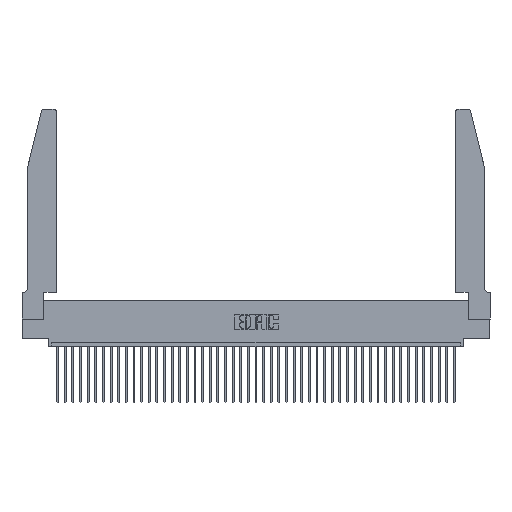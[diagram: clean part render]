
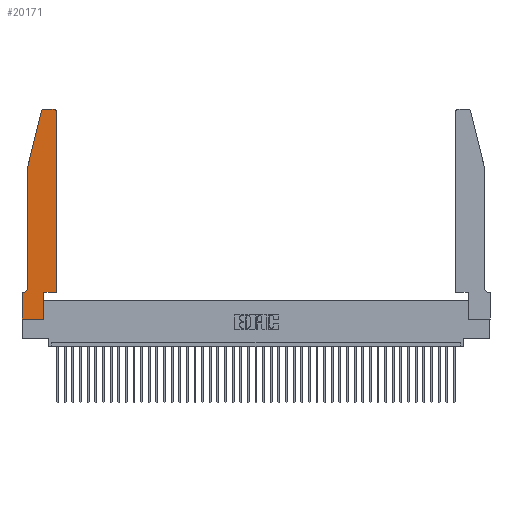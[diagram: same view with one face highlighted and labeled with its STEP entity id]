
A CAD part, top view. The second image highlights one B-rep face of the part: STEP entity #20171.
In plain terms, the highlighted planar face has unit normal (0, 0, 1).
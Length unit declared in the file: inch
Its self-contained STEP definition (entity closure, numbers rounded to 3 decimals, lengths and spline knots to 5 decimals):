
#223 = CARTESIAN_POINT ( 'NONE',  ( 0.4205, 2.72, 0.37 ) ) ;
#619 = AXIS2_PLACEMENT_3D ( 'NONE', #31257, #7567, #41190 ) ;
#623 = ORIENTED_EDGE ( 'NONE', *, *, #8489, .T. ) ;
#880 = CARTESIAN_POINT ( 'NONE',  ( 0.4505, 0.35, 0.37 ) ) ;
#1090 = ORIENTED_EDGE ( 'NONE', *, *, #26192, .T. ) ;
#1239 = CARTESIAN_POINT ( 'NONE',  ( 0.4205, 2.75, 0.37 ) ) ;
#1270 = CARTESIAN_POINT ( 'NONE',  ( 0.284, 2.75, 0.37 ) ) ;
#1503 = VERTEX_POINT ( 'NONE', #7037 ) ;
#1797 = DIRECTION ( 'NONE',  ( 0., 0., 1. ) ) ;
#5428 = LINE ( 'NONE', #5480, #12282 ) ;
#5480 = CARTESIAN_POINT ( 'NONE',  ( 0.4505, 0.35, 0.37 ) ) ;
#5614 = VERTEX_POINT ( 'NONE', #9768 ) ;
#6310 = ORIENTED_EDGE ( 'NONE', *, *, #35478, .T. ) ;
#6558 = LINE ( 'NONE', #9406, #32181 ) ;
#7037 = CARTESIAN_POINT ( 'NONE',  ( 0., 0.35, 0.37 ) ) ;
#7567 = DIRECTION ( 'NONE',  ( 0., 0., -1. ) ) ;
#8362 = VERTEX_POINT ( 'NONE', #10703 ) ;
#8384 = DIRECTION ( 'NONE',  ( 0., 1., 0. ) ) ;
#8489 = EDGE_CURVE ( 'NONE', #17175, #11979, #5428, .T. ) ;
#9182 = EDGE_CURVE ( 'NONE', #5614, #41324, #26899, .T. ) ;
#9406 = CARTESIAN_POINT ( 'NONE',  ( 0.0755, 2., 0.37 ) ) ;
#9527 = LINE ( 'NONE', #24423, #42977 ) ;
#9768 = CARTESIAN_POINT ( 'NONE',  ( 0., 0., 0.37 ) ) ;
#10390 = VERTEX_POINT ( 'NONE', #1270 ) ;
#10703 = CARTESIAN_POINT ( 'NONE',  ( 0.4505, 2.72, 0.37 ) ) ;
#11257 = AXIS2_PLACEMENT_3D ( 'NONE', #16678, #16818, #20434 ) ;
#11530 = CARTESIAN_POINT ( 'NONE',  ( 0.25487, 2.72718, 0.37 ) ) ;
#11979 = VERTEX_POINT ( 'NONE', #29067 ) ;
#12216 = EDGE_CURVE ( 'NONE', #32223, #40770, #21927, .T. ) ;
#12282 = VECTOR ( 'NONE', #39114, 39.37008 ) ;
#12546 = VERTEX_POINT ( 'NONE', #33564 ) ;
#12661 = VERTEX_POINT ( 'NONE', #1239 ) ;
#12969 = ORIENTED_EDGE ( 'NONE', *, *, #9182, .T. ) ;
#13023 = CARTESIAN_POINT ( 'NONE',  ( 0.0755, 2., 0.37 ) ) ;
#13304 = PLANE ( 'NONE',  #11257 ) ;
#13798 = VERTEX_POINT ( 'NONE', #11530 ) ;
#13979 = FACE_OUTER_BOUND ( 'NONE', #34819, .T. ) ;
#14500 = ORIENTED_EDGE ( 'NONE', *, *, #36134, .T. ) ;
#15165 = CARTESIAN_POINT ( 'NONE',  ( 0.2865, 0.35, 0.37 ) ) ;
#15218 = ORIENTED_EDGE ( 'NONE', *, *, #26518, .T. ) ;
#16555 = DIRECTION ( 'NONE',  ( 1., 0., 0. ) ) ;
#16678 = CARTESIAN_POINT ( 'NONE',  ( 0., 0.35, 0.37 ) ) ;
#16818 = DIRECTION ( 'NONE',  ( 0., 0., 1. ) ) ;
#16928 = LINE ( 'NONE', #13023, #32581 ) ;
#17175 = VERTEX_POINT ( 'NONE', #19725 ) ;
#18486 = ORIENTED_EDGE ( 'NONE', *, *, #12216, .T. ) ;
#18670 = EDGE_CURVE ( 'NONE', #10390, #13798, #35825, .T. ) ;
#19725 = CARTESIAN_POINT ( 'NONE',  ( 0.2865, 0.35, 0.37 ) ) ;
#20171 = ADVANCED_FACE ( 'NONE', ( #13979 ), #13304, .T. ) ;
#20434 = DIRECTION ( 'NONE',  ( 1., 0., 0. ) ) ;
#21247 = ORIENTED_EDGE ( 'NONE', *, *, #32891, .T. ) ;
#21551 = DIRECTION ( 'NONE',  ( 0., 1., 0. ) ) ;
#21913 = VECTOR ( 'NONE', #25814, 39.37008 ) ;
#21927 = CIRCLE ( 'NONE', #619, 0.07 ) ;
#22358 = EDGE_CURVE ( 'NONE', #1503, #5614, #9527, .T. ) ;
#22671 = CARTESIAN_POINT ( 'NONE',  ( 0.0755, 0.42, 0.37 ) ) ;
#22992 = LINE ( 'NONE', #38913, #21913 ) ;
#24009 = LINE ( 'NONE', #39280, #36523 ) ;
#24423 = CARTESIAN_POINT ( 'NONE',  ( 0., 0., 0.37 ) ) ;
#24719 = EDGE_CURVE ( 'NONE', #40770, #1503, #22992, .T. ) ;
#25194 = VECTOR ( 'NONE', #8384, 39.37008 ) ;
#25288 = DIRECTION ( 'NONE',  ( 1., 0., 0. ) ) ;
#25814 = DIRECTION ( 'NONE',  ( -1., 0., 0. ) ) ;
#26192 = EDGE_CURVE ( 'NONE', #8362, #12661, #26679, .T. ) ;
#26518 = EDGE_CURVE ( 'NONE', #12661, #10390, #24009, .T. ) ;
#26641 = DIRECTION ( 'NONE',  ( 0., 0., 1. ) ) ;
#26679 = CIRCLE ( 'NONE', #35533, 0.03 ) ;
#26899 = LINE ( 'NONE', #28851, #35159 ) ;
#28851 = CARTESIAN_POINT ( 'NONE',  ( 0., 0., 0.37 ) ) ;
#29067 = CARTESIAN_POINT ( 'NONE',  ( 0.4505, 0.35, 0.37 ) ) ;
#30878 = LINE ( 'NONE', #15165, #25194 ) ;
#31257 = CARTESIAN_POINT ( 'NONE',  ( 0.0055, 0.42, 0.37 ) ) ;
#31733 = DIRECTION ( 'NONE',  ( 1., 0., 0. ) ) ;
#31855 = ORIENTED_EDGE ( 'NONE', *, *, #18670, .T. ) ;
#32181 = VECTOR ( 'NONE', #35988, 39.37008 ) ;
#32223 = VERTEX_POINT ( 'NONE', #22671 ) ;
#32399 = CARTESIAN_POINT ( 'NONE',  ( 0.284, 2.72, 0.37 ) ) ;
#32581 = VECTOR ( 'NONE', #33417, 39.37008 ) ;
#32891 = EDGE_CURVE ( 'NONE', #12546, #32223, #6558, .T. ) ;
#33417 = DIRECTION ( 'NONE',  ( -0.239, -0.971, 0. ) ) ;
#33564 = CARTESIAN_POINT ( 'NONE',  ( 0.0755, 2., 0.37 ) ) ;
#33987 = ORIENTED_EDGE ( 'NONE', *, *, #22358, .T. ) ;
#34819 = EDGE_LOOP ( 'NONE', ( #15218, #31855, #41104, #21247, #18486, #41318, #33987, #12969, #6310, #623, #14500, #1090 ) ) ;
#35159 = VECTOR ( 'NONE', #31733, 39.37008 ) ;
#35478 = EDGE_CURVE ( 'NONE', #41324, #17175, #30878, .T. ) ;
#35533 = AXIS2_PLACEMENT_3D ( 'NONE', #223, #26641, #16555 ) ;
#35825 = CIRCLE ( 'NONE', #39730, 0.03 ) ;
#35988 = DIRECTION ( 'NONE',  ( 0., -1., 0. ) ) ;
#36134 = EDGE_CURVE ( 'NONE', #11979, #8362, #40248, .T. ) ;
#36347 = DIRECTION ( 'NONE',  ( -1., 0., 0. ) ) ;
#36523 = VECTOR ( 'NONE', #36347, 39.37008 ) ;
#36643 = CARTESIAN_POINT ( 'NONE',  ( 0.0055, 0.35, 0.37 ) ) ;
#37800 = DIRECTION ( 'NONE',  ( 0., -1., 0. ) ) ;
#38913 = CARTESIAN_POINT ( 'NONE',  ( 0.0755, 0.35, 0.37 ) ) ;
#39114 = DIRECTION ( 'NONE',  ( 1., 0., 0. ) ) ;
#39280 = CARTESIAN_POINT ( 'NONE',  ( 0.2605, 2.75, 0.37 ) ) ;
#39730 = AXIS2_PLACEMENT_3D ( 'NONE', #32399, #1797, #25288 ) ;
#40248 = LINE ( 'NONE', #880, #41263 ) ;
#40770 = VERTEX_POINT ( 'NONE', #36643 ) ;
#41104 = ORIENTED_EDGE ( 'NONE', *, *, #41429, .T. ) ;
#41190 = DIRECTION ( 'NONE',  ( -1., 0., 0. ) ) ;
#41263 = VECTOR ( 'NONE', #21551, 39.37008 ) ;
#41318 = ORIENTED_EDGE ( 'NONE', *, *, #24719, .T. ) ;
#41324 = VERTEX_POINT ( 'NONE', #42486 ) ;
#41429 = EDGE_CURVE ( 'NONE', #13798, #12546, #16928, .T. ) ;
#42486 = CARTESIAN_POINT ( 'NONE',  ( 0.2865, 0., 0.37 ) ) ;
#42977 = VECTOR ( 'NONE', #37800, 39.37008 ) ;
